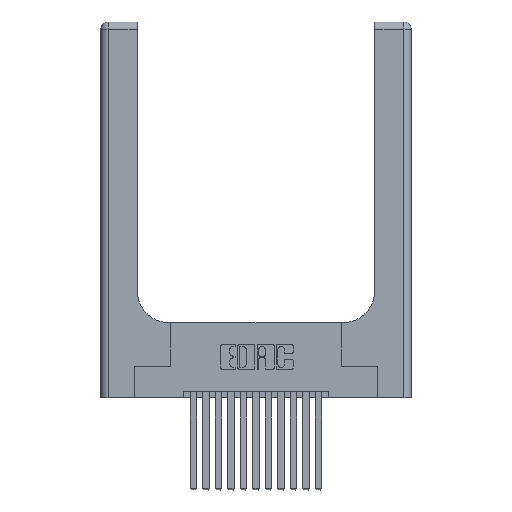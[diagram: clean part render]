
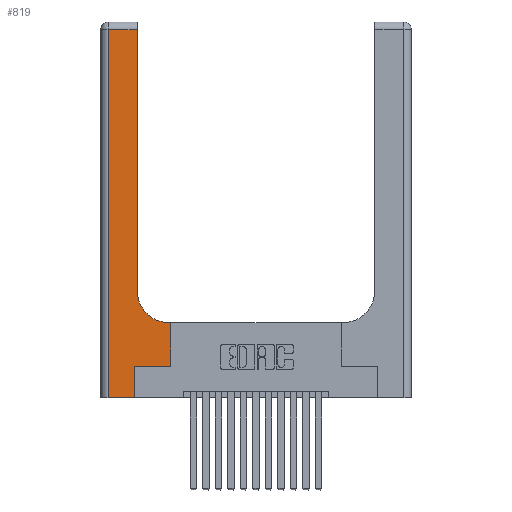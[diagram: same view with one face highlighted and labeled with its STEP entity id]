
A CAD part, top view. The second image highlights one B-rep face of the part: STEP entity #819.
In plain terms, the highlighted planar face has unit normal (0, 0, 1).
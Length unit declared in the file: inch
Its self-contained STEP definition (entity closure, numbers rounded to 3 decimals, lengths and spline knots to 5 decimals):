
#819 = ADVANCED_FACE ( 'NONE', ( #13434 ), #12253, .F. ) ;
#887 = EDGE_CURVE ( 'NONE', #16692, #4560, #12604, .T. ) ;
#955 = AXIS2_PLACEMENT_3D ( 'NONE', #12210, #12173, #12152 ) ;
#1150 = CARTESIAN_POINT ( 'NONE',  ( 0.06, 0., 0.37 ) ) ;
#1258 = VERTEX_POINT ( 'NONE', #5897 ) ;
#1496 = ORIENTED_EDGE ( 'NONE', *, *, #3057, .T. ) ;
#1567 = CARTESIAN_POINT ( 'NONE',  ( 0.269, 0.25, 0.37 ) ) ;
#1759 = VERTEX_POINT ( 'NONE', #16964 ) ;
#1973 = VECTOR ( 'NONE', #12669, 39.37008 ) ;
#2101 = VERTEX_POINT ( 'NONE', #1150 ) ;
#2170 = LINE ( 'NONE', #17601, #15937 ) ;
#2322 = EDGE_CURVE ( 'NONE', #1258, #7476, #5685, .T. ) ;
#2650 = CARTESIAN_POINT ( 'NONE',  ( 0.2915, 2.94, 0.37 ) ) ;
#3057 = EDGE_CURVE ( 'NONE', #6848, #1258, #14069, .T. ) ;
#3337 = EDGE_CURVE ( 'NONE', #2101, #6848, #13846, .T. ) ;
#3603 = CARTESIAN_POINT ( 'NONE',  ( 0.269, 0., 0.37 ) ) ;
#4153 = EDGE_CURVE ( 'NONE', #10372, #1759, #9582, .T. ) ;
#4353 = VERTEX_POINT ( 'NONE', #9148 ) ;
#4433 = CARTESIAN_POINT ( 'NONE',  ( 0.5415, 0.85, 0.37 ) ) ;
#4556 = DIRECTION ( 'NONE',  ( -1., 0., 0. ) ) ;
#4560 = VERTEX_POINT ( 'NONE', #10860 ) ;
#4682 = EDGE_CURVE ( 'NONE', #7476, #10372, #2170, .T. ) ;
#4843 = CARTESIAN_POINT ( 'NONE',  ( 0.06, 3., 0.37 ) ) ;
#4998 = LINE ( 'NONE', #7036, #15062 ) ;
#5040 = CIRCLE ( 'NONE', #16033, 0.25 ) ;
#5248 = VECTOR ( 'NONE', #7616, 39.37008 ) ;
#5640 = ORIENTED_EDGE ( 'NONE', *, *, #4682, .T. ) ;
#5685 = LINE ( 'NONE', #1567, #1973 ) ;
#5824 = DIRECTION ( 'NONE',  ( 1., 0., 0. ) ) ;
#5897 = CARTESIAN_POINT ( 'NONE',  ( 0.269, 0.25, 0.37 ) ) ;
#5996 = CARTESIAN_POINT ( 'NONE',  ( 0.269, 0., 0.37 ) ) ;
#6498 = ORIENTED_EDGE ( 'NONE', *, *, #12686, .T. ) ;
#6848 = VERTEX_POINT ( 'NONE', #5996 ) ;
#7036 = CARTESIAN_POINT ( 'NONE',  ( 0.2915, 3., 0.37 ) ) ;
#7251 = VECTOR ( 'NONE', #9129, 39.37008 ) ;
#7476 = VERTEX_POINT ( 'NONE', #17280 ) ;
#7616 = DIRECTION ( 'NONE',  ( 0., -1., 0. ) ) ;
#8923 = LINE ( 'NONE', #4843, #5248 ) ;
#9129 = DIRECTION ( 'NONE',  ( 0., 1., 0. ) ) ;
#9148 = CARTESIAN_POINT ( 'NONE',  ( 0.2915, 0.85, 0.37 ) ) ;
#9449 = DIRECTION ( 'NONE',  ( 0., 1., 0. ) ) ;
#9582 = LINE ( 'NONE', #16889, #13172 ) ;
#10372 = VERTEX_POINT ( 'NONE', #15475 ) ;
#10860 = CARTESIAN_POINT ( 'NONE',  ( 0.06, 2.94, 0.37 ) ) ;
#11242 = ORIENTED_EDGE ( 'NONE', *, *, #887, .T. ) ;
#11615 = DIRECTION ( 'NONE',  ( -1., 0., 0. ) ) ;
#11889 = CARTESIAN_POINT ( 'NONE',  ( 0., 2.94, 0.37 ) ) ;
#12079 = ORIENTED_EDGE ( 'NONE', *, *, #12906, .T. ) ;
#12152 = DIRECTION ( 'NONE',  ( -1., 0., 0. ) ) ;
#12171 = VECTOR ( 'NONE', #11615, 39.37008 ) ;
#12173 = DIRECTION ( 'NONE',  ( 0., 0., -1. ) ) ;
#12210 = CARTESIAN_POINT ( 'NONE',  ( 0., 3., 0.37 ) ) ;
#12253 = PLANE ( 'NONE',  #955 ) ;
#12604 = LINE ( 'NONE', #11889, #12171 ) ;
#12669 = DIRECTION ( 'NONE',  ( 1., 0., 0. ) ) ;
#12686 = EDGE_CURVE ( 'NONE', #1759, #4353, #5040, .T. ) ;
#12906 = EDGE_CURVE ( 'NONE', #4560, #2101, #8923, .T. ) ;
#13172 = VECTOR ( 'NONE', #4556, 39.37008 ) ;
#13434 = FACE_OUTER_BOUND ( 'NONE', #14900, .T. ) ;
#13684 = CARTESIAN_POINT ( 'NONE',  ( 0., 0., 0.37 ) ) ;
#13846 = LINE ( 'NONE', #13684, #17046 ) ;
#13953 = DIRECTION ( 'NONE',  ( 0., 1., 0. ) ) ;
#14014 = DIRECTION ( 'NONE',  ( 0., 0., -1. ) ) ;
#14069 = LINE ( 'NONE', #3603, #7251 ) ;
#14393 = ORIENTED_EDGE ( 'NONE', *, *, #16829, .T. ) ;
#14900 = EDGE_LOOP ( 'NONE', ( #14393, #11242, #12079, #15694, #1496, #16113, #5640, #16973, #6498 ) ) ;
#15062 = VECTOR ( 'NONE', #13953, 39.37008 ) ;
#15068 = DIRECTION ( 'NONE',  ( 1., 0., 0. ) ) ;
#15475 = CARTESIAN_POINT ( 'NONE',  ( 0.5585, 0.6, 0.37 ) ) ;
#15694 = ORIENTED_EDGE ( 'NONE', *, *, #3337, .T. ) ;
#15937 = VECTOR ( 'NONE', #9449, 39.37008 ) ;
#16033 = AXIS2_PLACEMENT_3D ( 'NONE', #4433, #14014, #5824 ) ;
#16113 = ORIENTED_EDGE ( 'NONE', *, *, #2322, .T. ) ;
#16692 = VERTEX_POINT ( 'NONE', #2650 ) ;
#16829 = EDGE_CURVE ( 'NONE', #4353, #16692, #4998, .T. ) ;
#16889 = CARTESIAN_POINT ( 'NONE',  ( 0.2915, 0.6, 0.37 ) ) ;
#16964 = CARTESIAN_POINT ( 'NONE',  ( 0.5415, 0.6, 0.37 ) ) ;
#16973 = ORIENTED_EDGE ( 'NONE', *, *, #4153, .T. ) ;
#17046 = VECTOR ( 'NONE', #15068, 39.37008 ) ;
#17280 = CARTESIAN_POINT ( 'NONE',  ( 0.5585, 0.25, 0.37 ) ) ;
#17601 = CARTESIAN_POINT ( 'NONE',  ( 0.5585, 0.25, 0.37 ) ) ;
